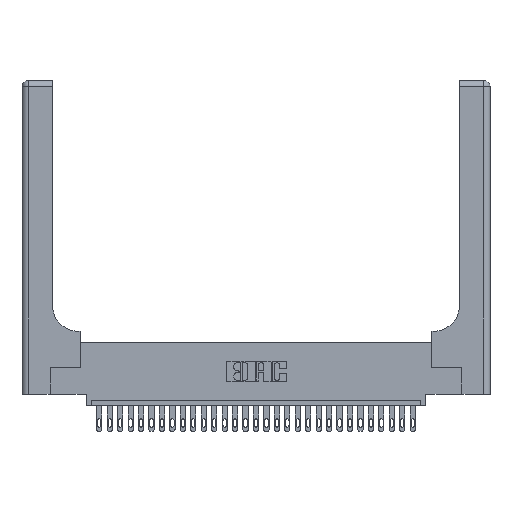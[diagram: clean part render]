
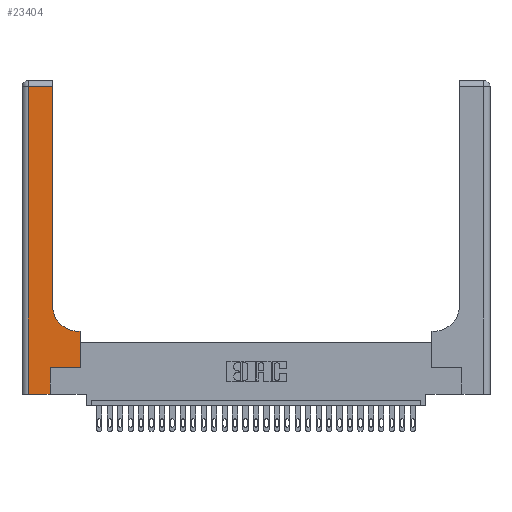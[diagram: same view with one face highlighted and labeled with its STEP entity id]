
A CAD part, top view. The second image highlights one B-rep face of the part: STEP entity #23404.
In plain terms, the highlighted planar face has unit normal (0, 0, 1).
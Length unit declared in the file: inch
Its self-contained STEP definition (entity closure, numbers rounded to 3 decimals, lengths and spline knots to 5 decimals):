
#562 = EDGE_LOOP ( 'NONE', ( #19527, #25336, #16394, #20858, #2687, #26358, #22524, #20344, #5010 ) ) ;
#699 = LINE ( 'NONE', #24564, #4717 ) ;
#946 = VECTOR ( 'NONE', #5769, 39.37008 ) ;
#2687 = ORIENTED_EDGE ( 'NONE', *, *, #5041, .T. ) ;
#3025 = CARTESIAN_POINT ( 'NONE',  ( 0.269, 0.25, 0.37 ) ) ;
#3346 = LINE ( 'NONE', #16289, #13488 ) ;
#3393 = DIRECTION ( 'NONE',  ( 0., 1., 0. ) ) ;
#4576 = EDGE_CURVE ( 'NONE', #29007, #9528, #9973, .T. ) ;
#4717 = VECTOR ( 'NONE', #3393, 39.37008 ) ;
#5010 = ORIENTED_EDGE ( 'NONE', *, *, #19905, .T. ) ;
#5041 = EDGE_CURVE ( 'NONE', #10732, #24004, #16218, .T. ) ;
#5360 = CARTESIAN_POINT ( 'NONE',  ( 0.5415, 0.6, 0.37 ) ) ;
#5494 = CARTESIAN_POINT ( 'NONE',  ( 0.269, 0., 0.37 ) ) ;
#5523 = DIRECTION ( 'NONE',  ( -1., 0., 0. ) ) ;
#5769 = DIRECTION ( 'NONE',  ( 0., 1., 0. ) ) ;
#6496 = EDGE_CURVE ( 'NONE', #10231, #29007, #10655, .T. ) ;
#8692 = CIRCLE ( 'NONE', #24556, 0.25 ) ;
#9528 = VERTEX_POINT ( 'NONE', #20680 ) ;
#9814 = CARTESIAN_POINT ( 'NONE',  ( 0.06, 2.94, 0.37 ) ) ;
#9868 = DIRECTION ( 'NONE',  ( 0., 0., -1. ) ) ;
#9911 = VECTOR ( 'NONE', #5523, 39.37008 ) ;
#9973 = LINE ( 'NONE', #23745, #19412 ) ;
#10082 = DIRECTION ( 'NONE',  ( 1., 0., 0. ) ) ;
#10231 = VERTEX_POINT ( 'NONE', #12566 ) ;
#10378 = CARTESIAN_POINT ( 'NONE',  ( 0.5585, 0.25, 0.37 ) ) ;
#10655 = LINE ( 'NONE', #19408, #9911 ) ;
#10732 = VERTEX_POINT ( 'NONE', #5494 ) ;
#11914 = EDGE_CURVE ( 'NONE', #13710, #10231, #699, .T. ) ;
#12566 = CARTESIAN_POINT ( 'NONE',  ( 0.2915, 2.94, 0.37 ) ) ;
#13103 = DIRECTION ( 'NONE',  ( 0., 1., 0. ) ) ;
#13488 = VECTOR ( 'NONE', #28110, 39.37008 ) ;
#13710 = VERTEX_POINT ( 'NONE', #14065 ) ;
#14038 = VECTOR ( 'NONE', #26943, 39.37008 ) ;
#14065 = CARTESIAN_POINT ( 'NONE',  ( 0.2915, 0.85, 0.37 ) ) ;
#14350 = VECTOR ( 'NONE', #13103, 39.37008 ) ;
#14736 = DIRECTION ( 'NONE',  ( -1., 0., 0. ) ) ;
#15602 = CARTESIAN_POINT ( 'NONE',  ( 0.2915, 0.6, 0.37 ) ) ;
#16218 = LINE ( 'NONE', #17196, #946 ) ;
#16289 = CARTESIAN_POINT ( 'NONE',  ( 0., 0., 0.37 ) ) ;
#16394 = ORIENTED_EDGE ( 'NONE', *, *, #4576, .T. ) ;
#16482 = LINE ( 'NONE', #17635, #17222 ) ;
#17196 = CARTESIAN_POINT ( 'NONE',  ( 0.269, 0., 0.37 ) ) ;
#17222 = VECTOR ( 'NONE', #17425, 39.37008 ) ;
#17425 = DIRECTION ( 'NONE',  ( 1., 0., 0. ) ) ;
#17635 = CARTESIAN_POINT ( 'NONE',  ( 0.269, 0.25, 0.37 ) ) ;
#17804 = CARTESIAN_POINT ( 'NONE',  ( 0.5585, 0.6, 0.37 ) ) ;
#18998 = CARTESIAN_POINT ( 'NONE',  ( 0., 3., 0.37 ) ) ;
#19408 = CARTESIAN_POINT ( 'NONE',  ( 0., 2.94, 0.37 ) ) ;
#19412 = VECTOR ( 'NONE', #21503, 39.37008 ) ;
#19422 = LINE ( 'NONE', #27164, #14350 ) ;
#19527 = ORIENTED_EDGE ( 'NONE', *, *, #11914, .T. ) ;
#19623 = VERTEX_POINT ( 'NONE', #17804 ) ;
#19810 = DIRECTION ( 'NONE',  ( 0., 0., -1. ) ) ;
#19905 = EDGE_CURVE ( 'NONE', #25818, #13710, #8692, .T. ) ;
#20344 = ORIENTED_EDGE ( 'NONE', *, *, #25443, .T. ) ;
#20680 = CARTESIAN_POINT ( 'NONE',  ( 0.06, 0., 0.37 ) ) ;
#20858 = ORIENTED_EDGE ( 'NONE', *, *, #28907, .T. ) ;
#21503 = DIRECTION ( 'NONE',  ( 0., -1., 0. ) ) ;
#21624 = LINE ( 'NONE', #15602, #14038 ) ;
#21910 = CARTESIAN_POINT ( 'NONE',  ( 0.5415, 0.85, 0.37 ) ) ;
#21915 = VERTEX_POINT ( 'NONE', #10378 ) ;
#21999 = AXIS2_PLACEMENT_3D ( 'NONE', #18998, #9868, #14736 ) ;
#22013 = EDGE_CURVE ( 'NONE', #21915, #19623, #19422, .T. ) ;
#22490 = EDGE_CURVE ( 'NONE', #24004, #21915, #16482, .T. ) ;
#22524 = ORIENTED_EDGE ( 'NONE', *, *, #22013, .T. ) ;
#23404 = ADVANCED_FACE ( 'NONE', ( #25839 ), #28374, .F. ) ;
#23745 = CARTESIAN_POINT ( 'NONE',  ( 0.06, 3., 0.37 ) ) ;
#24004 = VERTEX_POINT ( 'NONE', #3025 ) ;
#24556 = AXIS2_PLACEMENT_3D ( 'NONE', #21910, #19810, #10082 ) ;
#24564 = CARTESIAN_POINT ( 'NONE',  ( 0.2915, 3., 0.37 ) ) ;
#25336 = ORIENTED_EDGE ( 'NONE', *, *, #6496, .T. ) ;
#25443 = EDGE_CURVE ( 'NONE', #19623, #25818, #21624, .T. ) ;
#25818 = VERTEX_POINT ( 'NONE', #5360 ) ;
#25839 = FACE_OUTER_BOUND ( 'NONE', #562, .T. ) ;
#26358 = ORIENTED_EDGE ( 'NONE', *, *, #22490, .T. ) ;
#26943 = DIRECTION ( 'NONE',  ( -1., 0., 0. ) ) ;
#27164 = CARTESIAN_POINT ( 'NONE',  ( 0.5585, 0.25, 0.37 ) ) ;
#28110 = DIRECTION ( 'NONE',  ( 1., 0., 0. ) ) ;
#28374 = PLANE ( 'NONE',  #21999 ) ;
#28907 = EDGE_CURVE ( 'NONE', #9528, #10732, #3346, .T. ) ;
#29007 = VERTEX_POINT ( 'NONE', #9814 ) ;
